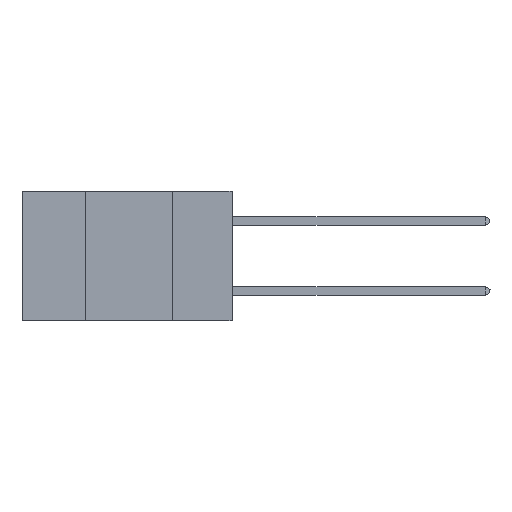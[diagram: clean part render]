
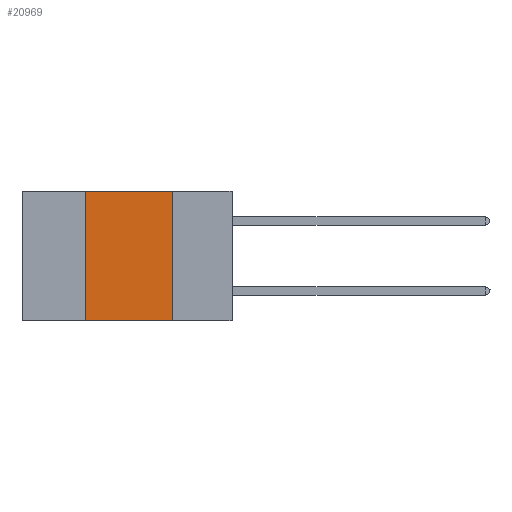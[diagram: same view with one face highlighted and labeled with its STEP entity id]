
A CAD part, left-side view. The second image highlights one B-rep face of the part: STEP entity #20969.
In plain terms, the highlighted planar face has unit normal (-1, 0, 0).
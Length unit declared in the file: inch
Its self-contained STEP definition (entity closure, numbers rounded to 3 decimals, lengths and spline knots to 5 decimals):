
#137 = EDGE_LOOP ( 'NONE', ( #12952, #8138, #3402, #21406 ) ) ;
#495 = LINE ( 'NONE', #23090, #5393 ) ;
#1469 = LINE ( 'NONE', #14748, #9509 ) ;
#2751 = CARTESIAN_POINT ( 'NONE',  ( 0., 0.17, -0.37 ) ) ;
#3402 = ORIENTED_EDGE ( 'NONE', *, *, #7353, .F. ) ;
#4998 = VERTEX_POINT ( 'NONE', #8653 ) ;
#5393 = VECTOR ( 'NONE', #17189, 39.37008 ) ;
#5853 = CARTESIAN_POINT ( 'NONE',  ( 0., 0.42, 0. ) ) ;
#6053 = CARTESIAN_POINT ( 'NONE',  ( 0., 0.17, 0. ) ) ;
#6514 = VECTOR ( 'NONE', #31784, 39.37008 ) ;
#7353 = EDGE_CURVE ( 'NONE', #13692, #4998, #18665, .T. ) ;
#8138 = ORIENTED_EDGE ( 'NONE', *, *, #9321, .F. ) ;
#8653 = CARTESIAN_POINT ( 'NONE',  ( 0., 0.42, 0. ) ) ;
#9321 = EDGE_CURVE ( 'NONE', #4998, #17089, #495, .T. ) ;
#9509 = VECTOR ( 'NONE', #30237, 39.37008 ) ;
#12001 = DIRECTION ( 'NONE',  ( 0., 0., 1. ) ) ;
#12168 = CARTESIAN_POINT ( 'NONE',  ( 0., 0.6, 0. ) ) ;
#12403 = PLANE ( 'NONE',  #12576 ) ;
#12576 = AXIS2_PLACEMENT_3D ( 'NONE', #12168, #22439, #24982 ) ;
#12952 = ORIENTED_EDGE ( 'NONE', *, *, #22548, .F. ) ;
#13692 = VERTEX_POINT ( 'NONE', #18945 ) ;
#14748 = CARTESIAN_POINT ( 'NONE',  ( 0., 0.17, 0. ) ) ;
#16104 = EDGE_CURVE ( 'NONE', #13692, #26635, #26870, .T. ) ;
#17089 = VERTEX_POINT ( 'NONE', #6053 ) ;
#17189 = DIRECTION ( 'NONE',  ( 0., -1., 0. ) ) ;
#18665 = LINE ( 'NONE', #5853, #24691 ) ;
#18945 = CARTESIAN_POINT ( 'NONE',  ( 0., 0.42, -0.37 ) ) ;
#20969 = ADVANCED_FACE ( 'NONE', ( #23161 ), #12403, .F. ) ;
#21406 = ORIENTED_EDGE ( 'NONE', *, *, #16104, .T. ) ;
#22439 = DIRECTION ( 'NONE',  ( 1., 0., 0. ) ) ;
#22548 = EDGE_CURVE ( 'NONE', #17089, #26635, #1469, .T. ) ;
#23090 = CARTESIAN_POINT ( 'NONE',  ( 0., 0.6, 0. ) ) ;
#23161 = FACE_OUTER_BOUND ( 'NONE', #137, .T. ) ;
#24691 = VECTOR ( 'NONE', #12001, 39.37008 ) ;
#24982 = DIRECTION ( 'NONE',  ( 0., 0., -1. ) ) ;
#26635 = VERTEX_POINT ( 'NONE', #2751 ) ;
#26870 = LINE ( 'NONE', #29197, #6514 ) ;
#29197 = CARTESIAN_POINT ( 'NONE',  ( 0., 0.6, -0.37 ) ) ;
#30237 = DIRECTION ( 'NONE',  ( 0., 0., -1. ) ) ;
#31784 = DIRECTION ( 'NONE',  ( 0., -1., 0. ) ) ;
